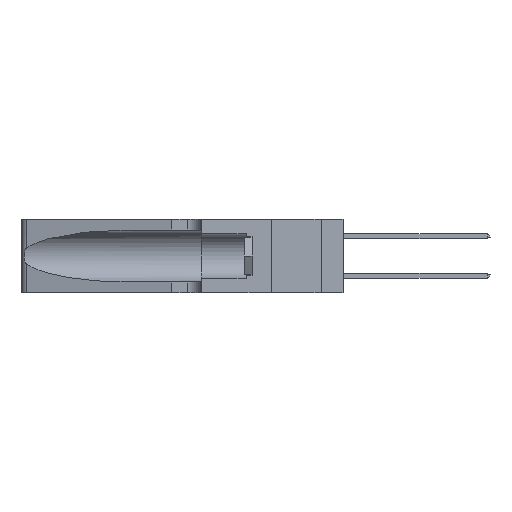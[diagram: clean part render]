
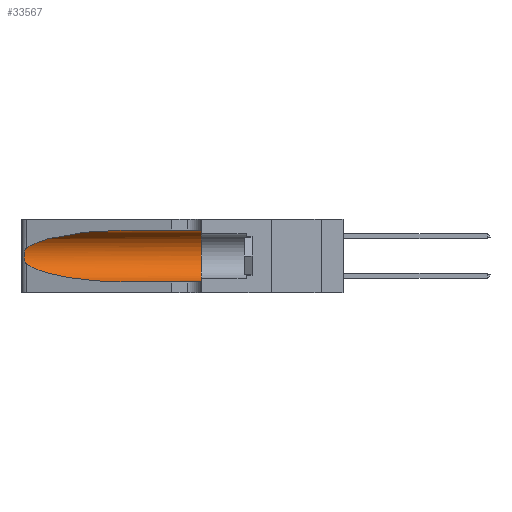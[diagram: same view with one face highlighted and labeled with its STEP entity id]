
A CAD part, left-side view. The second image highlights one B-rep face of the part: STEP entity #33567.
In plain terms, the highlighted cylindrical face has radius 3.308 mm (diameter 6.617 mm), a partial arc.
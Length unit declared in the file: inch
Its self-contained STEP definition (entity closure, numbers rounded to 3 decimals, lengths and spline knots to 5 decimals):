
#2152 = FACE_OUTER_BOUND ( 'NONE', #7567, .T. ) ;
#2193 = VERTEX_POINT ( 'NONE', #23855 ) ;
#2494 = CARTESIAN_POINT ( 'NONE',  ( 0.26017, 1.23833, 0.17102 ) ) ;
#2901 = AXIS2_PLACEMENT_3D ( 'NONE', #21855, #4307, #24788 ) ;
#3504 = EDGE_CURVE ( 'NONE', #2193, #8900, #31821, .T. ) ;
#4307 = DIRECTION ( 'NONE',  ( 0., 1., 0. ) ) ;
#5484 = CARTESIAN_POINT ( 'NONE',  ( 0.25789, 1.23486, 0.15765 ) ) ;
#5786 = CARTESIAN_POINT ( 'NONE',  ( 0.2373, 1.15595, 0.08982 ) ) ;
#5972 = CARTESIAN_POINT ( 'NONE',  ( 0.25487, 1.22718, 0.22369 ) ) ;
#5989 = EDGE_CURVE ( 'NONE', #18593, #29815, #8365, .T. ) ;
#6522 = VERTEX_POINT ( 'NONE', #26155 ) ;
#7463 = VECTOR ( 'NONE', #29380, 39.37008 ) ;
#7567 = EDGE_LOOP ( 'NONE', ( #10389, #29629, #23046, #20227, #30917, #26976 ) ) ;
#8302 = CARTESIAN_POINT ( 'NONE',  ( 0.25487, 1.22718, 0.22369 ) ) ;
#8365 = LINE ( 'NONE', #9582, #7463 ) ;
#8424 = CARTESIAN_POINT ( 'NONE',  ( 0.25555, 1.22993, 0.14849 ) ) ;
#8900 = VERTEX_POINT ( 'NONE', #15741 ) ;
#9056 = CYLINDRICAL_SURFACE ( 'NONE', #23947, 0.13025 ) ;
#9394 = EDGE_CURVE ( 'NONE', #2193, #30970, #30741, .T. ) ;
#9582 = CARTESIAN_POINT ( 'NONE',  ( 0.1305, 1.61858, 0.05475 ) ) ;
#10389 = ORIENTED_EDGE ( 'NONE', *, *, #9394, .T. ) ;
#11260 = CARTESIAN_POINT ( 'NONE',  ( 0.25555, 1.22994, 0.2215 ) ) ;
#11689 = CARTESIAN_POINT ( 'NONE',  ( 0.1305, 0.72297, 0.05475 ) ) ;
#11880 = EDGE_CURVE ( 'NONE', #8900, #29815, #17254, .T. ) ;
#12727 =( BOUNDED_CURVE ( )  B_SPLINE_CURVE ( 3, ( #34877, #5786, #29156, #11689 ),
 .UNSPECIFIED., .F., .T. ) 
 B_SPLINE_CURVE_WITH_KNOTS ( ( 4, 4 ),
 ( 3.44316, 4.71239 ),
 .UNSPECIFIED. ) 
 CURVE ( )  GEOMETRIC_REPRESENTATION_ITEM ( )  RATIONAL_B_SPLINE_CURVE ( ( 1., 0.87, 0.87, 1. ) ) 
 REPRESENTATION_ITEM ( '' )  );
#14203 = CARTESIAN_POINT ( 'NONE',  ( 0.25787, 1.23484, 0.2124 ) ) ;
#15335 = CARTESIAN_POINT ( 'NONE',  ( 0.1305, 1.61858, 0.31525 ) ) ;
#15741 = CARTESIAN_POINT ( 'NONE',  ( 0.1305, 0.35, 0.31525 ) ) ;
#16131 = B_SPLINE_CURVE_WITH_KNOTS ( 'NONE', 3,
 ( #8302, #11260, #31679, #14203, #34585, #17153, #37465, #20061, #2494, #23008, #5484, #25923, #8424, #28850 ),
 .UNSPECIFIED., .F., .F.,
 ( 4, 2, 2, 2, 2, 2, 4 ),
 ( 0., 0.00027, 0.00053, 0.00107, 0.0016, 0.00187, 0.00214 ),
 .UNSPECIFIED. ) ;
#16298 = DIRECTION ( 'NONE',  ( 0., 0., -1. ) ) ;
#17153 = CARTESIAN_POINT ( 'NONE',  ( 0.26018, 1.23835, 0.19895 ) ) ;
#17254 = CIRCLE ( 'NONE', #2901, 0.13025 ) ;
#17637 = CARTESIAN_POINT ( 'NONE',  ( 0.18966, 0.96281, 0.31525 ) ) ;
#18593 = VERTEX_POINT ( 'NONE', #36383 ) ;
#19111 = DIRECTION ( 'NONE',  ( 0., -1., 0. ) ) ;
#20061 = CARTESIAN_POINT ( 'NONE',  ( 0.26075, 1.23896, 0.178 ) ) ;
#20227 = ORIENTED_EDGE ( 'NONE', *, *, #5989, .T. ) ;
#20614 = CARTESIAN_POINT ( 'NONE',  ( 0.1305, 0.72297, 0.31525 ) ) ;
#21855 = CARTESIAN_POINT ( 'NONE',  ( 0.1305, 0.35, 0.185 ) ) ;
#23008 = CARTESIAN_POINT ( 'NONE',  ( 0.25856, 1.23593, 0.16098 ) ) ;
#23046 = ORIENTED_EDGE ( 'NONE', *, *, #27651, .T. ) ;
#23511 = CARTESIAN_POINT ( 'NONE',  ( 0.2373, 1.15595, 0.28018 ) ) ;
#23855 = CARTESIAN_POINT ( 'NONE',  ( 0.1305, 0.72297, 0.31525 ) ) ;
#23947 = AXIS2_PLACEMENT_3D ( 'NONE', #33758, #19111, #16298 ) ;
#24788 = DIRECTION ( 'NONE',  ( 0., 0., 1. ) ) ;
#25923 = CARTESIAN_POINT ( 'NONE',  ( 0.25639, 1.23186, 0.15144 ) ) ;
#26155 = CARTESIAN_POINT ( 'NONE',  ( 0.25487, 1.22718, 0.14631 ) ) ;
#26279 = CARTESIAN_POINT ( 'NONE',  ( 0.1305, 0.35, 0.05475 ) ) ;
#26942 = DIRECTION ( 'NONE',  ( 0., -1., 0. ) ) ;
#26976 = ORIENTED_EDGE ( 'NONE', *, *, #3504, .F. ) ;
#27651 = EDGE_CURVE ( 'NONE', #6522, #18593, #12727, .T. ) ;
#28194 = EDGE_CURVE ( 'NONE', #30970, #6522, #16131, .T. ) ;
#28850 = CARTESIAN_POINT ( 'NONE',  ( 0.25487, 1.22718, 0.14631 ) ) ;
#29156 = CARTESIAN_POINT ( 'NONE',  ( 0.18966, 0.96281, 0.05475 ) ) ;
#29380 = DIRECTION ( 'NONE',  ( 0., -1., 0. ) ) ;
#29629 = ORIENTED_EDGE ( 'NONE', *, *, #28194, .T. ) ;
#29815 = VERTEX_POINT ( 'NONE', #26279 ) ;
#29984 = VECTOR ( 'NONE', #26942, 39.37008 ) ;
#30741 =( BOUNDED_CURVE ( )  B_SPLINE_CURVE ( 3, ( #20614, #17637, #23511, #5972 ),
 .UNSPECIFIED., .F., .T. ) 
 B_SPLINE_CURVE_WITH_KNOTS ( ( 4, 4 ),
 ( 1.5708, 2.84003 ),
 .UNSPECIFIED. ) 
 CURVE ( )  GEOMETRIC_REPRESENTATION_ITEM ( )  RATIONAL_B_SPLINE_CURVE ( ( 1., 0.87, 0.87, 1. ) ) 
 REPRESENTATION_ITEM ( '' )  );
#30917 = ORIENTED_EDGE ( 'NONE', *, *, #11880, .F. ) ;
#30970 = VERTEX_POINT ( 'NONE', #31838 ) ;
#31679 = CARTESIAN_POINT ( 'NONE',  ( 0.25639, 1.23184, 0.21858 ) ) ;
#31821 = LINE ( 'NONE', #15335, #29984 ) ;
#31838 = CARTESIAN_POINT ( 'NONE',  ( 0.25487, 1.22718, 0.22369 ) ) ;
#33567 = ADVANCED_FACE ( 'NONE', ( #2152 ), #9056, .F. ) ;
#33758 = CARTESIAN_POINT ( 'NONE',  ( 0.1305, 1.61858, 0.185 ) ) ;
#34585 = CARTESIAN_POINT ( 'NONE',  ( 0.25854, 1.2359, 0.20912 ) ) ;
#34877 = CARTESIAN_POINT ( 'NONE',  ( 0.25487, 1.22718, 0.14631 ) ) ;
#36383 = CARTESIAN_POINT ( 'NONE',  ( 0.1305, 0.72297, 0.05475 ) ) ;
#37465 = CARTESIAN_POINT ( 'NONE',  ( 0.26075, 1.23896, 0.19203 ) ) ;
